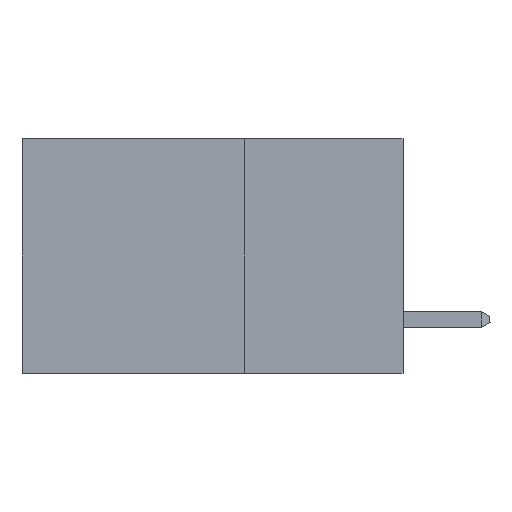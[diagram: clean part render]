
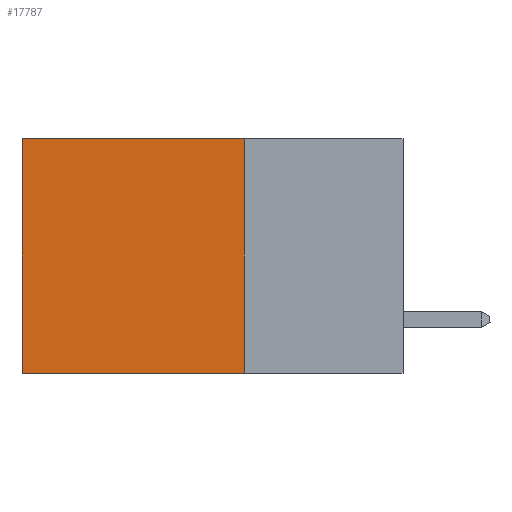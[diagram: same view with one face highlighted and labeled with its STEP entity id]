
A CAD part, left-side view. The second image highlights one B-rep face of the part: STEP entity #17787.
In plain terms, the highlighted planar face has unit normal (-1, 0, 0).
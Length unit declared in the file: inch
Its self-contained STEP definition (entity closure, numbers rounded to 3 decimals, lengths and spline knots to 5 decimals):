
#524 = VECTOR ( 'NONE', #14197, 39.37008 ) ;
#1794 = VECTOR ( 'NONE', #10695, 39.37008 ) ;
#2492 = EDGE_CURVE ( 'NONE', #24298, #14422, #9354, .T. ) ;
#3067 = ORIENTED_EDGE ( 'NONE', *, *, #20163, .T. ) ;
#4423 = DIRECTION ( 'NONE',  ( 0., 1., 0. ) ) ;
#6507 = CARTESIAN_POINT ( 'NONE',  ( 0.2875, 0.25, 0. ) ) ;
#6682 = CARTESIAN_POINT ( 'NONE',  ( 0.2875, 0.25, 0. ) ) ;
#7101 = LINE ( 'NONE', #14018, #524 ) ;
#8199 = CARTESIAN_POINT ( 'NONE',  ( 0.2875, 0.6, -0.37 ) ) ;
#8458 = CARTESIAN_POINT ( 'NONE',  ( 0.2875, 0.25, 0. ) ) ;
#9354 = LINE ( 'NONE', #16889, #1794 ) ;
#10492 = LINE ( 'NONE', #16321, #13968 ) ;
#10695 = DIRECTION ( 'NONE',  ( 0., 1., 0. ) ) ;
#11281 = LINE ( 'NONE', #6682, #19780 ) ;
#11668 = EDGE_CURVE ( 'NONE', #20156, #24298, #7101, .T. ) ;
#13202 = ORIENTED_EDGE ( 'NONE', *, *, #11668, .F. ) ;
#13334 = DIRECTION ( 'NONE',  ( 0., 0., -1. ) ) ;
#13604 = ORIENTED_EDGE ( 'NONE', *, *, #2492, .F. ) ;
#13776 = ORIENTED_EDGE ( 'NONE', *, *, #23945, .T. ) ;
#13968 = VECTOR ( 'NONE', #18684, 39.37008 ) ;
#14018 = CARTESIAN_POINT ( 'NONE',  ( 0.2875, 0.25, 0. ) ) ;
#14197 = DIRECTION ( 'NONE',  ( 0., 0., -1. ) ) ;
#14322 = PLANE ( 'NONE',  #24250 ) ;
#14422 = VERTEX_POINT ( 'NONE', #8199 ) ;
#15536 = VERTEX_POINT ( 'NONE', #24015 ) ;
#16321 = CARTESIAN_POINT ( 'NONE',  ( 0.2875, 0.6, 0. ) ) ;
#16889 = CARTESIAN_POINT ( 'NONE',  ( 0.2875, 0.25, -0.37 ) ) ;
#17787 = ADVANCED_FACE ( 'NONE', ( #26044 ), #14322, .F. ) ;
#18684 = DIRECTION ( 'NONE',  ( 0., 0., -1. ) ) ;
#19780 = VECTOR ( 'NONE', #4423, 39.37008 ) ;
#20156 = VERTEX_POINT ( 'NONE', #6507 ) ;
#20163 = EDGE_CURVE ( 'NONE', #15536, #14422, #10492, .T. ) ;
#21849 = EDGE_LOOP ( 'NONE', ( #3067, #13604, #13202, #13776 ) ) ;
#22079 = CARTESIAN_POINT ( 'NONE',  ( 0.2875, 0.25, -0.37 ) ) ;
#22553 = DIRECTION ( 'NONE',  ( 1., 0., 0. ) ) ;
#23945 = EDGE_CURVE ( 'NONE', #20156, #15536, #11281, .T. ) ;
#24015 = CARTESIAN_POINT ( 'NONE',  ( 0.2875, 0.6, 0. ) ) ;
#24250 = AXIS2_PLACEMENT_3D ( 'NONE', #8458, #22553, #13334 ) ;
#24298 = VERTEX_POINT ( 'NONE', #22079 ) ;
#26044 = FACE_OUTER_BOUND ( 'NONE', #21849, .T. ) ;
